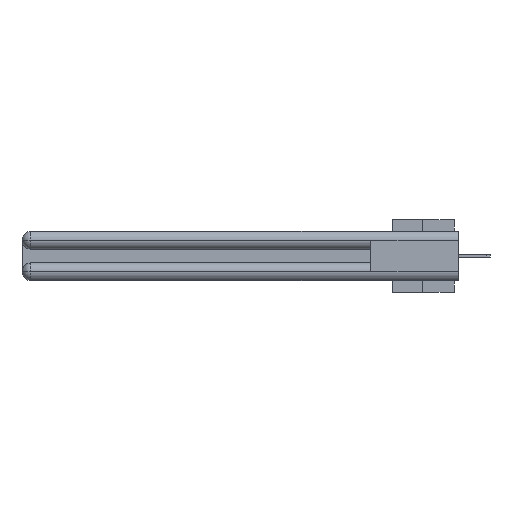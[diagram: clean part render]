
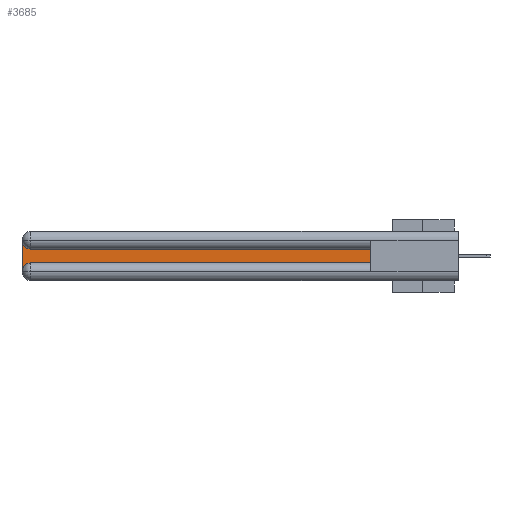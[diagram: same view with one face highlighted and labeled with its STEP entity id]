
A CAD part, left-side view. The second image highlights one B-rep face of the part: STEP entity #3685.
In plain terms, the highlighted planar face has unit normal (-1, 0, 0).
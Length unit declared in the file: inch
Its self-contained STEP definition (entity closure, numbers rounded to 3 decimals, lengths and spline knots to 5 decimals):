
#693 = CARTESIAN_POINT ( 'NONE',  ( 0.075, 3., -0.1225 ) ) ;
#1665 = ORIENTED_EDGE ( 'NONE', *, *, #7401, .T. ) ;
#1936 = LINE ( 'NONE', #22304, #18691 ) ;
#2492 = ORIENTED_EDGE ( 'NONE', *, *, #4236, .T. ) ;
#3276 = ORIENTED_EDGE ( 'NONE', *, *, #31709, .T. ) ;
#3685 = ADVANCED_FACE ( 'NONE', ( #23355 ), #25097, .F. ) ;
#3837 = VERTEX_POINT ( 'NONE', #18230 ) ;
#4236 = EDGE_CURVE ( 'NONE', #3837, #16487, #1936, .T. ) ;
#5401 = CARTESIAN_POINT ( 'NONE',  ( 0.075, 2.94, -0.0625 ) ) ;
#6064 = VERTEX_POINT ( 'NONE', #10088 ) ;
#6644 = CARTESIAN_POINT ( 'NONE',  ( 0.075, 0.6, -0.2175 ) ) ;
#7265 = VERTEX_POINT ( 'NONE', #24718 ) ;
#7394 = CARTESIAN_POINT ( 'NONE',  ( 0.075, 2.94, -0.1225 ) ) ;
#7401 = EDGE_CURVE ( 'NONE', #22259, #6064, #29239, .T. ) ;
#7910 = DIRECTION ( 'NONE',  ( 0., 0., -1. ) ) ;
#8065 = CARTESIAN_POINT ( 'NONE',  ( 0.075, 2.94, -0.2775 ) ) ;
#8354 = ORIENTED_EDGE ( 'NONE', *, *, #17672, .T. ) ;
#9153 = CIRCLE ( 'NONE', #31716, 0.06 ) ;
#9165 = ORIENTED_EDGE ( 'NONE', *, *, #14123, .T. ) ;
#9185 = DIRECTION ( 'NONE',  ( 0., 0., 1. ) ) ;
#9852 = CARTESIAN_POINT ( 'NONE',  ( 0.075, 0.6, -0.2175 ) ) ;
#10038 = DIRECTION ( 'NONE',  ( 0., 0., -1. ) ) ;
#10088 = CARTESIAN_POINT ( 'NONE',  ( 0.075, 2.94, -0.2175 ) ) ;
#10570 = DIRECTION ( 'NONE',  ( 0., 0., -1. ) ) ;
#11305 = LINE ( 'NONE', #6644, #23669 ) ;
#13831 = CARTESIAN_POINT ( 'NONE',  ( 0.075, 3., -0.2175 ) ) ;
#14123 = EDGE_CURVE ( 'NONE', #16487, #7265, #9153, .T. ) ;
#14485 = VECTOR ( 'NONE', #24643, 39.37008 ) ;
#15761 = CARTESIAN_POINT ( 'NONE',  ( 0.075, 3., -0.2775 ) ) ;
#16487 = VERTEX_POINT ( 'NONE', #7394 ) ;
#17187 = DIRECTION ( 'NONE',  ( 1., 0., 0. ) ) ;
#17672 = EDGE_CURVE ( 'NONE', #6064, #25252, #21014, .T. ) ;
#18230 = CARTESIAN_POINT ( 'NONE',  ( 0.075, 0.6, -0.1225 ) ) ;
#18691 = VECTOR ( 'NONE', #24763, 39.37008 ) ;
#21014 = LINE ( 'NONE', #9852, #14485 ) ;
#21090 = AXIS2_PLACEMENT_3D ( 'NONE', #8065, #25339, #10570 ) ;
#21776 = EDGE_CURVE ( 'NONE', #7265, #22259, #29994, .T. ) ;
#22259 = VERTEX_POINT ( 'NONE', #15761 ) ;
#22304 = CARTESIAN_POINT ( 'NONE',  ( 0.075, 0.6, -0.1225 ) ) ;
#22744 = DIRECTION ( 'NONE',  ( 1., 0., 0. ) ) ;
#23355 = FACE_OUTER_BOUND ( 'NONE', #32072, .T. ) ;
#23466 = VECTOR ( 'NONE', #30997, 39.37008 ) ;
#23669 = VECTOR ( 'NONE', #9185, 39.37008 ) ;
#24643 = DIRECTION ( 'NONE',  ( 0., -1., 0. ) ) ;
#24718 = CARTESIAN_POINT ( 'NONE',  ( 0.075, 3., -0.0625 ) ) ;
#24763 = DIRECTION ( 'NONE',  ( 0., 1., 0. ) ) ;
#25097 = PLANE ( 'NONE',  #32102 ) ;
#25252 = VERTEX_POINT ( 'NONE', #26627 ) ;
#25339 = DIRECTION ( 'NONE',  ( 1., 0., 0. ) ) ;
#26627 = CARTESIAN_POINT ( 'NONE',  ( 0.075, 0.6, -0.2175 ) ) ;
#29239 = CIRCLE ( 'NONE', #21090, 0.06 ) ;
#29994 = LINE ( 'NONE', #13831, #23466 ) ;
#30395 = ORIENTED_EDGE ( 'NONE', *, *, #21776, .T. ) ;
#30997 = DIRECTION ( 'NONE',  ( 0., 0., -1. ) ) ;
#31709 = EDGE_CURVE ( 'NONE', #25252, #3837, #11305, .T. ) ;
#31716 = AXIS2_PLACEMENT_3D ( 'NONE', #5401, #22744, #7910 ) ;
#32072 = EDGE_LOOP ( 'NONE', ( #2492, #9165, #30395, #1665, #8354, #3276 ) ) ;
#32102 = AXIS2_PLACEMENT_3D ( 'NONE', #693, #17187, #10038 ) ;
